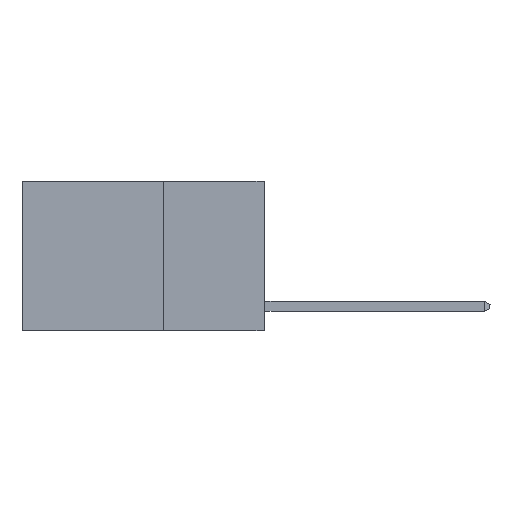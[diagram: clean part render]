
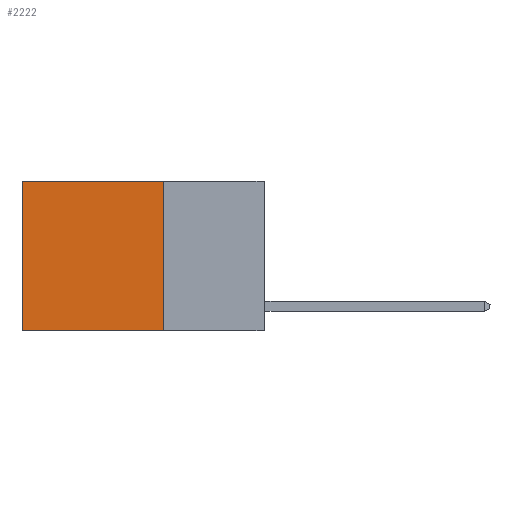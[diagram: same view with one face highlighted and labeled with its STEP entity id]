
A CAD part, left-side view. The second image highlights one B-rep face of the part: STEP entity #2222.
In plain terms, the highlighted planar face has unit normal (-1, 0, 0).
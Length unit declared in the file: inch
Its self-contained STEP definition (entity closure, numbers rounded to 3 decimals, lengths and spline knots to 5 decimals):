
#191 = DIRECTION ( 'NONE',  ( 1., 0., 0. ) ) ;
#498 = VECTOR ( 'NONE', #2392, 39.37008 ) ;
#1264 = LINE ( 'NONE', #9152, #498 ) ;
#2128 = ORIENTED_EDGE ( 'NONE', *, *, #4962, .F. ) ;
#2222 = ADVANCED_FACE ( 'NONE', ( #8306 ), #3789, .F. ) ;
#2392 = DIRECTION ( 'NONE',  ( 0., 1., 0. ) ) ;
#3192 = VECTOR ( 'NONE', #7891, 39.37008 ) ;
#3789 = PLANE ( 'NONE',  #9011 ) ;
#3942 = CARTESIAN_POINT ( 'NONE',  ( 0.2625, 0.25, 0. ) ) ;
#3957 = VECTOR ( 'NONE', #11257, 39.37008 ) ;
#4310 = EDGE_LOOP ( 'NONE', ( #14824, #8888, #2128, #8534 ) ) ;
#4962 = EDGE_CURVE ( 'NONE', #6782, #14560, #11069, .T. ) ;
#5856 = EDGE_CURVE ( 'NONE', #14560, #8770, #1264, .T. ) ;
#6508 = CARTESIAN_POINT ( 'NONE',  ( 0.2625, 0.25, 0. ) ) ;
#6782 = VERTEX_POINT ( 'NONE', #3942 ) ;
#7378 = VECTOR ( 'NONE', #14368, 39.37008 ) ;
#7488 = CARTESIAN_POINT ( 'NONE',  ( 0.2625, 0.25, -0.37 ) ) ;
#7891 = DIRECTION ( 'NONE',  ( 0., 0., -1. ) ) ;
#8093 = VERTEX_POINT ( 'NONE', #13114 ) ;
#8306 = FACE_OUTER_BOUND ( 'NONE', #4310, .T. ) ;
#8376 = CARTESIAN_POINT ( 'NONE',  ( 0.2625, 0.25, 0. ) ) ;
#8534 = ORIENTED_EDGE ( 'NONE', *, *, #12060, .T. ) ;
#8770 = VERTEX_POINT ( 'NONE', #13760 ) ;
#8888 = ORIENTED_EDGE ( 'NONE', *, *, #5856, .F. ) ;
#9011 = AXIS2_PLACEMENT_3D ( 'NONE', #8376, #191, #13996 ) ;
#9152 = CARTESIAN_POINT ( 'NONE',  ( 0.2625, 0.25, -0.37 ) ) ;
#10144 = CARTESIAN_POINT ( 'NONE',  ( 0.2625, 0.6, 0. ) ) ;
#10458 = EDGE_CURVE ( 'NONE', #8093, #8770, #13603, .T. ) ;
#11069 = LINE ( 'NONE', #13178, #7378 ) ;
#11257 = DIRECTION ( 'NONE',  ( 0., 1., 0. ) ) ;
#12060 = EDGE_CURVE ( 'NONE', #6782, #8093, #12535, .T. ) ;
#12535 = LINE ( 'NONE', #6508, #3957 ) ;
#13114 = CARTESIAN_POINT ( 'NONE',  ( 0.2625, 0.6, 0. ) ) ;
#13178 = CARTESIAN_POINT ( 'NONE',  ( 0.2625, 0.25, 0. ) ) ;
#13603 = LINE ( 'NONE', #10144, #3192 ) ;
#13760 = CARTESIAN_POINT ( 'NONE',  ( 0.2625, 0.6, -0.37 ) ) ;
#13996 = DIRECTION ( 'NONE',  ( 0., 0., -1. ) ) ;
#14368 = DIRECTION ( 'NONE',  ( 0., 0., -1. ) ) ;
#14560 = VERTEX_POINT ( 'NONE', #7488 ) ;
#14824 = ORIENTED_EDGE ( 'NONE', *, *, #10458, .T. ) ;
